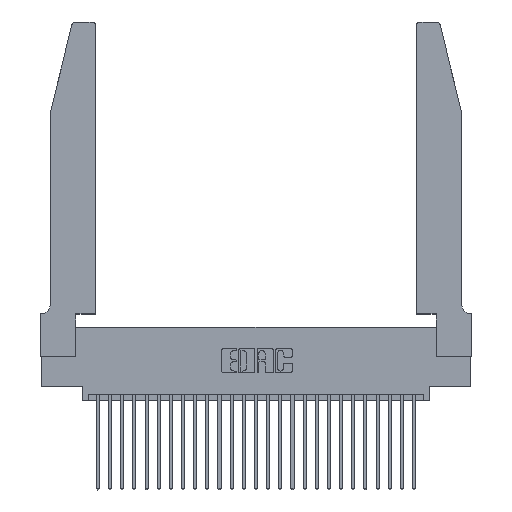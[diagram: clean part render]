
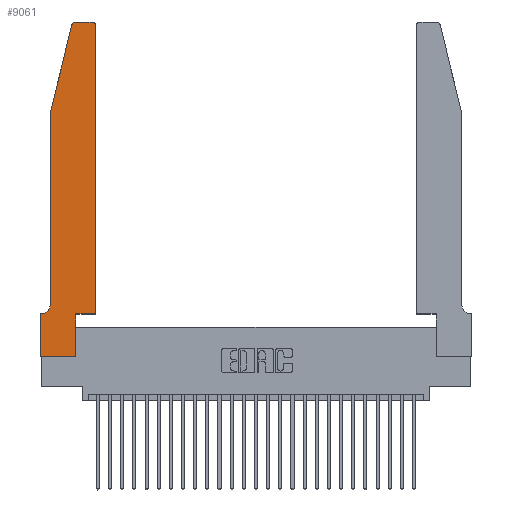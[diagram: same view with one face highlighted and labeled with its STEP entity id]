
A CAD part, top view. The second image highlights one B-rep face of the part: STEP entity #9061.
In plain terms, the highlighted planar face has unit normal (0, 0, 1).
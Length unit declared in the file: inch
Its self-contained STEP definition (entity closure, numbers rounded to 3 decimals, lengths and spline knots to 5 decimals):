
#89 = VECTOR ( 'NONE', #12022, 39.37008 ) ;
#692 = ORIENTED_EDGE ( 'NONE', *, *, #19174, .T. ) ;
#1424 = LINE ( 'NONE', #22667, #19057 ) ;
#1600 = EDGE_CURVE ( 'NONE', #11517, #14897, #1424, .T. ) ;
#1853 = LINE ( 'NONE', #8853, #11685 ) ;
#2077 = AXIS2_PLACEMENT_3D ( 'NONE', #22660, #9598, #24840 ) ;
#2193 = ORIENTED_EDGE ( 'NONE', *, *, #27090, .T. ) ;
#2459 = EDGE_CURVE ( 'NONE', #9833, #20468, #15092, .T. ) ;
#3335 = EDGE_CURVE ( 'NONE', #14161, #19128, #18762, .T. ) ;
#3664 = ORIENTED_EDGE ( 'NONE', *, *, #12483, .T. ) ;
#3951 = CARTESIAN_POINT ( 'NONE',  ( 0.2865, 0., 0.37 ) ) ;
#4066 = VECTOR ( 'NONE', #11504, 39.37008 ) ;
#4141 = AXIS2_PLACEMENT_3D ( 'NONE', #22094, #16204, #12689 ) ;
#4338 = ORIENTED_EDGE ( 'NONE', *, *, #1600, .T. ) ;
#4926 = AXIS2_PLACEMENT_3D ( 'NONE', #13598, #22089, #24292 ) ;
#5130 = ORIENTED_EDGE ( 'NONE', *, *, #9186, .T. ) ;
#5495 = EDGE_CURVE ( 'NONE', #13078, #22614, #6454, .T. ) ;
#6014 = CARTESIAN_POINT ( 'NONE',  ( 0.25487, 2.72718, 0.37 ) ) ;
#6454 = CIRCLE ( 'NONE', #4141, 0.03 ) ;
#6928 = EDGE_LOOP ( 'NONE', ( #2193, #19874, #9650, #21708, #3664, #25153, #5130, #15766, #4338, #13835, #17572, #692 ) ) ;
#7807 = DIRECTION ( 'NONE',  ( 1., 0., 0. ) ) ;
#8414 = DIRECTION ( 'NONE',  ( 1., 0., 0. ) ) ;
#8617 = EDGE_CURVE ( 'NONE', #25679, #11517, #13398, .T. ) ;
#8853 = CARTESIAN_POINT ( 'NONE',  ( 0.2605, 2.75, 0.37 ) ) ;
#8955 = CARTESIAN_POINT ( 'NONE',  ( 0.4505, 0.35, 0.37 ) ) ;
#8977 = VECTOR ( 'NONE', #12189, 39.37008 ) ;
#9061 = ADVANCED_FACE ( 'NONE', ( #26311 ), #20176, .T. ) ;
#9186 = EDGE_CURVE ( 'NONE', #9644, #25679, #14038, .T. ) ;
#9504 = CARTESIAN_POINT ( 'NONE',  ( 0.4505, 2.72, 0.37 ) ) ;
#9598 = DIRECTION ( 'NONE',  ( 0., 0., 1. ) ) ;
#9644 = VERTEX_POINT ( 'NONE', #20027 ) ;
#9650 = ORIENTED_EDGE ( 'NONE', *, *, #21649, .T. ) ;
#9655 = CIRCLE ( 'NONE', #2077, 0.03 ) ;
#9833 = VERTEX_POINT ( 'NONE', #25020 ) ;
#9852 = CARTESIAN_POINT ( 'NONE',  ( 0.0755, 2., 0.37 ) ) ;
#9947 = DIRECTION ( 'NONE',  ( -0.239, -0.971, 0. ) ) ;
#10187 = CARTESIAN_POINT ( 'NONE',  ( 0.0755, 2., 0.37 ) ) ;
#10350 = CARTESIAN_POINT ( 'NONE',  ( 0., 0., 0.37 ) ) ;
#10721 = CARTESIAN_POINT ( 'NONE',  ( 0.284, 2.75, 0.37 ) ) ;
#11504 = DIRECTION ( 'NONE',  ( -1., 0., 0. ) ) ;
#11517 = VERTEX_POINT ( 'NONE', #3951 ) ;
#11685 = VECTOR ( 'NONE', #15500, 39.37008 ) ;
#11924 = CARTESIAN_POINT ( 'NONE',  ( 0.4505, 0.35, 0.37 ) ) ;
#12022 = DIRECTION ( 'NONE',  ( 0., 1., 0. ) ) ;
#12189 = DIRECTION ( 'NONE',  ( 0., -1., 0. ) ) ;
#12332 = VERTEX_POINT ( 'NONE', #26531 ) ;
#12483 = EDGE_CURVE ( 'NONE', #20468, #12332, #24490, .T. ) ;
#12689 = DIRECTION ( 'NONE',  ( 1., 0., 0. ) ) ;
#13078 = VERTEX_POINT ( 'NONE', #10721 ) ;
#13398 = LINE ( 'NONE', #18731, #18504 ) ;
#13598 = CARTESIAN_POINT ( 'NONE',  ( 0., 0.35, 0.37 ) ) ;
#13835 = ORIENTED_EDGE ( 'NONE', *, *, #23962, .T. ) ;
#13905 = DIRECTION ( 'NONE',  ( 0., 1., 0. ) ) ;
#13974 = VECTOR ( 'NONE', #9947, 39.37008 ) ;
#14038 = LINE ( 'NONE', #10350, #25638 ) ;
#14161 = VERTEX_POINT ( 'NONE', #8955 ) ;
#14716 = DIRECTION ( 'NONE',  ( 0., -1., 0. ) ) ;
#14897 = VERTEX_POINT ( 'NONE', #26492 ) ;
#15092 = LINE ( 'NONE', #10187, #8977 ) ;
#15500 = DIRECTION ( 'NONE',  ( -1., 0., 0. ) ) ;
#15766 = ORIENTED_EDGE ( 'NONE', *, *, #8617, .T. ) ;
#16204 = DIRECTION ( 'NONE',  ( 0., 0., 1. ) ) ;
#16556 = CARTESIAN_POINT ( 'NONE',  ( 0.0755, 0.42, 0.37 ) ) ;
#17572 = ORIENTED_EDGE ( 'NONE', *, *, #3335, .T. ) ;
#17946 = CARTESIAN_POINT ( 'NONE',  ( 0.0755, 0.35, 0.37 ) ) ;
#18504 = VECTOR ( 'NONE', #7807, 39.37008 ) ;
#18731 = CARTESIAN_POINT ( 'NONE',  ( 0., 0., 0.37 ) ) ;
#18762 = LINE ( 'NONE', #11924, #89 ) ;
#19057 = VECTOR ( 'NONE', #13905, 39.37008 ) ;
#19128 = VERTEX_POINT ( 'NONE', #9504 ) ;
#19174 = EDGE_CURVE ( 'NONE', #19128, #22462, #9655, .T. ) ;
#19260 = CARTESIAN_POINT ( 'NONE',  ( 0.4505, 0.35, 0.37 ) ) ;
#19757 = AXIS2_PLACEMENT_3D ( 'NONE', #27797, #21365, #25840 ) ;
#19874 = ORIENTED_EDGE ( 'NONE', *, *, #5495, .T. ) ;
#20027 = CARTESIAN_POINT ( 'NONE',  ( 0., 0.35, 0.37 ) ) ;
#20176 = PLANE ( 'NONE',  #4926 ) ;
#20468 = VERTEX_POINT ( 'NONE', #16556 ) ;
#20671 = CARTESIAN_POINT ( 'NONE',  ( 0.4205, 2.75, 0.37 ) ) ;
#21115 = LINE ( 'NONE', #17946, #4066 ) ;
#21365 = DIRECTION ( 'NONE',  ( 0., 0., -1. ) ) ;
#21649 = EDGE_CURVE ( 'NONE', #22614, #9833, #25559, .T. ) ;
#21708 = ORIENTED_EDGE ( 'NONE', *, *, #2459, .T. ) ;
#22089 = DIRECTION ( 'NONE',  ( 0., 0., 1. ) ) ;
#22094 = CARTESIAN_POINT ( 'NONE',  ( 0.284, 2.72, 0.37 ) ) ;
#22462 = VERTEX_POINT ( 'NONE', #20671 ) ;
#22614 = VERTEX_POINT ( 'NONE', #6014 ) ;
#22660 = CARTESIAN_POINT ( 'NONE',  ( 0.4205, 2.72, 0.37 ) ) ;
#22667 = CARTESIAN_POINT ( 'NONE',  ( 0.2865, 0.35, 0.37 ) ) ;
#22920 = EDGE_CURVE ( 'NONE', #12332, #9644, #21115, .T. ) ;
#23099 = LINE ( 'NONE', #19260, #25136 ) ;
#23962 = EDGE_CURVE ( 'NONE', #14897, #14161, #23099, .T. ) ;
#24292 = DIRECTION ( 'NONE',  ( 1., 0., 0. ) ) ;
#24490 = CIRCLE ( 'NONE', #19757, 0.07 ) ;
#24840 = DIRECTION ( 'NONE',  ( 1., 0., 0. ) ) ;
#25020 = CARTESIAN_POINT ( 'NONE',  ( 0.0755, 2., 0.37 ) ) ;
#25136 = VECTOR ( 'NONE', #8414, 39.37008 ) ;
#25153 = ORIENTED_EDGE ( 'NONE', *, *, #22920, .T. ) ;
#25559 = LINE ( 'NONE', #9852, #13974 ) ;
#25579 = CARTESIAN_POINT ( 'NONE',  ( 0., 0., 0.37 ) ) ;
#25638 = VECTOR ( 'NONE', #14716, 39.37008 ) ;
#25679 = VERTEX_POINT ( 'NONE', #25579 ) ;
#25840 = DIRECTION ( 'NONE',  ( -1., 0., 0. ) ) ;
#26311 = FACE_OUTER_BOUND ( 'NONE', #6928, .T. ) ;
#26492 = CARTESIAN_POINT ( 'NONE',  ( 0.2865, 0.35, 0.37 ) ) ;
#26531 = CARTESIAN_POINT ( 'NONE',  ( 0.0055, 0.35, 0.37 ) ) ;
#27090 = EDGE_CURVE ( 'NONE', #22462, #13078, #1853, .T. ) ;
#27797 = CARTESIAN_POINT ( 'NONE',  ( 0.0055, 0.42, 0.37 ) ) ;
